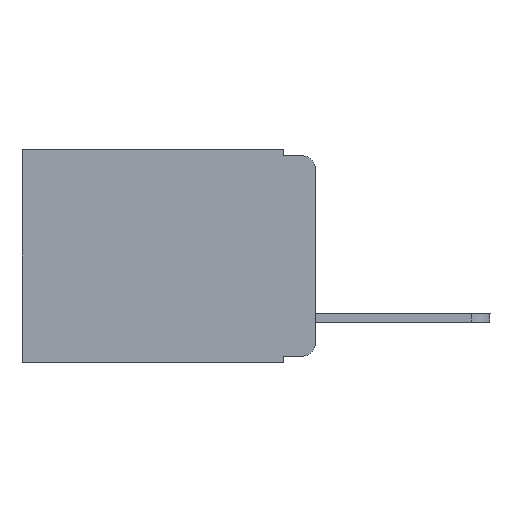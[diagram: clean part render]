
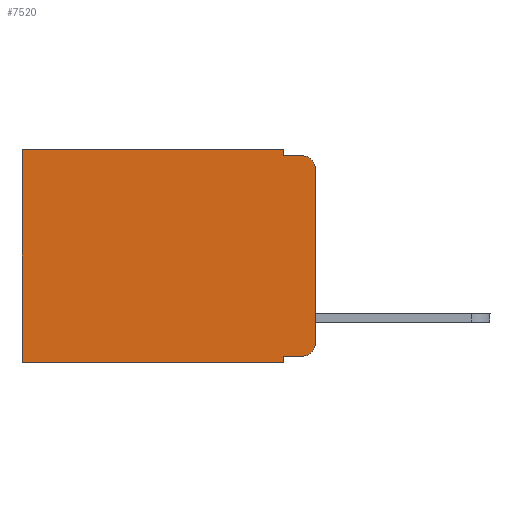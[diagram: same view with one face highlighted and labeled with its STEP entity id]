
A CAD part, left-side view. The second image highlights one B-rep face of the part: STEP entity #7520.
In plain terms, the highlighted planar face has unit normal (-1, 0, 0).
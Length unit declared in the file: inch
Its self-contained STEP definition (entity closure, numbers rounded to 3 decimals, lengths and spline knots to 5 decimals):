
#171 = EDGE_CURVE ( 'NONE', #4938, #5293, #15446, .T. ) ;
#236 = CARTESIAN_POINT ( 'NONE',  ( 0.298, 0.051, -0.01 ) ) ;
#312 = ORIENTED_EDGE ( 'NONE', *, *, #9317, .T. ) ;
#1527 = LINE ( 'NONE', #22334, #11182 ) ;
#1863 = EDGE_CURVE ( 'NONE', #17974, #19532, #10269, .T. ) ;
#1965 = VECTOR ( 'NONE', #15797, 39.37008 ) ;
#3338 = VECTOR ( 'NONE', #13460, 39.37008 ) ;
#4014 = EDGE_CURVE ( 'NONE', #15042, #4938, #16431, .T. ) ;
#4476 = LINE ( 'NONE', #6399, #15623 ) ;
#4662 = VERTEX_POINT ( 'NONE', #11907 ) ;
#4938 = VERTEX_POINT ( 'NONE', #8820 ) ;
#5186 = ORIENTED_EDGE ( 'NONE', *, *, #171, .F. ) ;
#5284 = EDGE_CURVE ( 'NONE', #8738, #19532, #1527, .T. ) ;
#5291 = VERTEX_POINT ( 'NONE', #236 ) ;
#5293 = VERTEX_POINT ( 'NONE', #6764 ) ;
#5814 = FACE_OUTER_BOUND ( 'NONE', #16585, .T. ) ;
#6389 = LINE ( 'NONE', #16410, #3338 ) ;
#6399 = CARTESIAN_POINT ( 'NONE',  ( 0.298, 0.473, 0. ) ) ;
#6453 = ORIENTED_EDGE ( 'NONE', *, *, #4014, .F. ) ;
#6513 = DIRECTION ( 'NONE',  ( 0., 0., -1. ) ) ;
#6668 = ORIENTED_EDGE ( 'NONE', *, *, #12085, .T. ) ;
#6764 = CARTESIAN_POINT ( 'NONE',  ( 0.298, 0.473, -0.343 ) ) ;
#6876 = DIRECTION ( 'NONE',  ( 0., 0., -1. ) ) ;
#6991 = DIRECTION ( 'NONE',  ( -1., 0., 0. ) ) ;
#7520 = ADVANCED_FACE ( 'NONE', ( #5814 ), #12781, .F. ) ;
#7554 = EDGE_CURVE ( 'NONE', #15761, #5291, #6389, .T. ) ;
#8105 = LINE ( 'NONE', #16968, #20268 ) ;
#8271 = CARTESIAN_POINT ( 'NONE',  ( 0.298, 0., -0.03 ) ) ;
#8341 = VECTOR ( 'NONE', #11497, 39.37008 ) ;
#8738 = VERTEX_POINT ( 'NONE', #8271 ) ;
#8820 = CARTESIAN_POINT ( 'NONE',  ( 0.298, 0.051, -0.343 ) ) ;
#9276 = ORIENTED_EDGE ( 'NONE', *, *, #5284, .F. ) ;
#9317 = EDGE_CURVE ( 'NONE', #8738, #14899, #11419, .T. ) ;
#9414 = VECTOR ( 'NONE', #16709, 39.37008 ) ;
#9896 = CARTESIAN_POINT ( 'NONE',  ( 0.298, 0., 0. ) ) ;
#10269 = CIRCLE ( 'NONE', #15057, 0.02 ) ;
#10736 = DIRECTION ( 'NONE',  ( 1., 0., 0. ) ) ;
#10826 = EDGE_CURVE ( 'NONE', #5291, #14899, #8105, .T. ) ;
#10851 = DIRECTION ( 'NONE',  ( 0., 0., -1. ) ) ;
#10924 = CARTESIAN_POINT ( 'NONE',  ( 0.298, 0.051, -0.333 ) ) ;
#11069 = CARTESIAN_POINT ( 'NONE',  ( 0.298, 0.02, -0.01 ) ) ;
#11182 = VECTOR ( 'NONE', #6876, 39.37008 ) ;
#11419 = CIRCLE ( 'NONE', #20811, 0.02 ) ;
#11497 = DIRECTION ( 'NONE',  ( 0., 1., 0. ) ) ;
#11907 = CARTESIAN_POINT ( 'NONE',  ( 0.298, 0.473, 0. ) ) ;
#12085 = EDGE_CURVE ( 'NONE', #15042, #17974, #12398, .T. ) ;
#12110 = DIRECTION ( 'NONE',  ( 0., 0., -1. ) ) ;
#12398 = LINE ( 'NONE', #10924, #1965 ) ;
#12781 = PLANE ( 'NONE',  #19969 ) ;
#12887 = CARTESIAN_POINT ( 'NONE',  ( 0.298, 0.02, -0.333 ) ) ;
#13197 = LINE ( 'NONE', #9896, #8341 ) ;
#13460 = DIRECTION ( 'NONE',  ( 0., 0., -1. ) ) ;
#14100 = CARTESIAN_POINT ( 'NONE',  ( 0.298, 0.051, 0. ) ) ;
#14217 = ORIENTED_EDGE ( 'NONE', *, *, #1863, .T. ) ;
#14899 = VERTEX_POINT ( 'NONE', #11069 ) ;
#15042 = VERTEX_POINT ( 'NONE', #18770 ) ;
#15057 = AXIS2_PLACEMENT_3D ( 'NONE', #21688, #15126, #16477 ) ;
#15126 = DIRECTION ( 'NONE',  ( -1., 0., 0. ) ) ;
#15183 = CARTESIAN_POINT ( 'NONE',  ( 0.298, 0.051, 0. ) ) ;
#15446 = LINE ( 'NONE', #17034, #9414 ) ;
#15623 = VECTOR ( 'NONE', #6513, 39.37008 ) ;
#15761 = VERTEX_POINT ( 'NONE', #14100 ) ;
#15797 = DIRECTION ( 'NONE',  ( 0., -1., 0. ) ) ;
#15916 = ORIENTED_EDGE ( 'NONE', *, *, #18645, .T. ) ;
#16071 = VECTOR ( 'NONE', #21866, 39.37008 ) ;
#16410 = CARTESIAN_POINT ( 'NONE',  ( 0.298, 0.051, 0. ) ) ;
#16431 = LINE ( 'NONE', #15183, #16071 ) ;
#16477 = DIRECTION ( 'NONE',  ( 0., 0., -1. ) ) ;
#16585 = EDGE_LOOP ( 'NONE', ( #9276, #312, #18336, #20417, #15916, #21953, #5186, #6453, #6668, #14217 ) ) ;
#16709 = DIRECTION ( 'NONE',  ( 0., 1., 0. ) ) ;
#16968 = CARTESIAN_POINT ( 'NONE',  ( 0.298, 0.051, -0.01 ) ) ;
#17034 = CARTESIAN_POINT ( 'NONE',  ( 0.298, 0., -0.343 ) ) ;
#17974 = VERTEX_POINT ( 'NONE', #12887 ) ;
#17998 = CARTESIAN_POINT ( 'NONE',  ( 0.298, 0., 0. ) ) ;
#18336 = ORIENTED_EDGE ( 'NONE', *, *, #10826, .F. ) ;
#18645 = EDGE_CURVE ( 'NONE', #15761, #4662, #13197, .T. ) ;
#18770 = CARTESIAN_POINT ( 'NONE',  ( 0.298, 0.051, -0.333 ) ) ;
#19531 = EDGE_CURVE ( 'NONE', #4662, #5293, #4476, .T. ) ;
#19532 = VERTEX_POINT ( 'NONE', #20249 ) ;
#19969 = AXIS2_PLACEMENT_3D ( 'NONE', #17998, #10736, #10851 ) ;
#20249 = CARTESIAN_POINT ( 'NONE',  ( 0.298, 0., -0.313 ) ) ;
#20268 = VECTOR ( 'NONE', #21963, 39.37008 ) ;
#20417 = ORIENTED_EDGE ( 'NONE', *, *, #7554, .F. ) ;
#20723 = CARTESIAN_POINT ( 'NONE',  ( 0.298, 0.02, -0.03 ) ) ;
#20811 = AXIS2_PLACEMENT_3D ( 'NONE', #20723, #6991, #12110 ) ;
#21688 = CARTESIAN_POINT ( 'NONE',  ( 0.298, 0.02, -0.313 ) ) ;
#21866 = DIRECTION ( 'NONE',  ( 0., 0., -1. ) ) ;
#21953 = ORIENTED_EDGE ( 'NONE', *, *, #19531, .T. ) ;
#21963 = DIRECTION ( 'NONE',  ( 0., -1., 0. ) ) ;
#22334 = CARTESIAN_POINT ( 'NONE',  ( 0.298, 0., 0. ) ) ;
